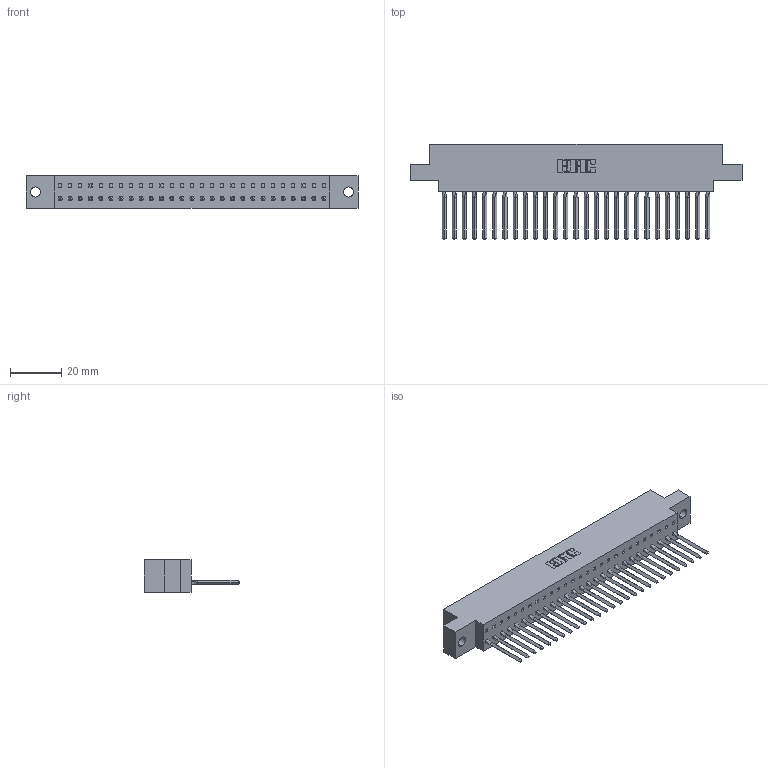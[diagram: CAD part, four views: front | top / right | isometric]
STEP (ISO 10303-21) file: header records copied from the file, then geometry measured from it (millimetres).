
FILE_DESCRIPTION (( 'STEP AP203' ), '1' );
FILE_NAME ('317-027-541-604.STEP', '2020-02-27T19:14:55', ( '' ), ( '' ), 'SwSTEP 2.0', 'SolidWorks 2016', '' );
FILE_SCHEMA (( 'CONFIG_CONTROL_DESIGN' ));
Length unit declared in the file: inch
Products named in the file (3): 317-027-541-604; 317 Part_.156 Dia - TH; 317-290-002_541
Assembly tree (28 placements, depth 2):
  317-027-541-604
    317 Part_.156 Dia - TH
    317-290-002_541  x27
Bounding box: 129.69 x 37.34 x 12.7 mm (x, y, z)
Volume: 20482.7 mm3; surface area: 28261.3 mm2
Topology: 28 solids, 28 shells, 4206 faces, 11993 edges, 7796 vertices
Faces by surface type: plane 3406, cylinder 692, bspline 108
Entity records: 41808 total; most frequent: CARTESIAN_POINT 8066, ORIENTED_EDGE 7346, DIRECTION 6023, EDGE_CURVE 3673, LINE 3309, VECTOR 3309, VERTEX_POINT 2440, AXIS2_PLACEMENT_3D 1357
